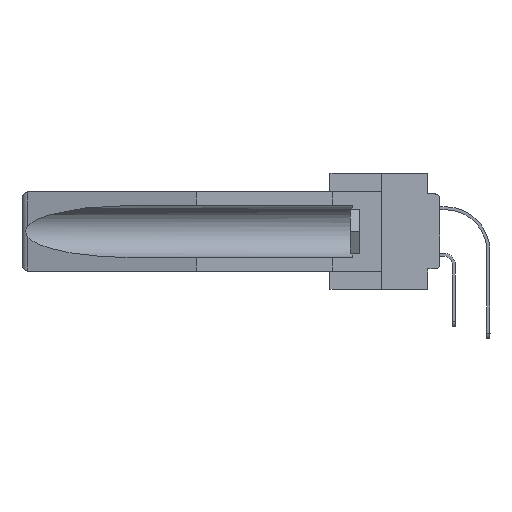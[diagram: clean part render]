
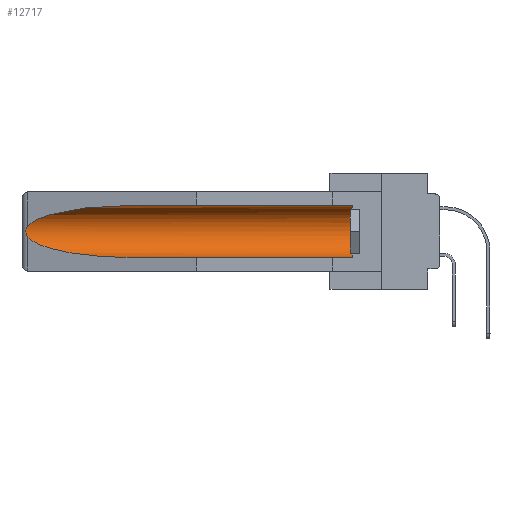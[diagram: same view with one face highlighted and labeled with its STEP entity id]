
A CAD part, left-side view. The second image highlights one B-rep face of the part: STEP entity #12717.
In plain terms, the highlighted cylindrical face has radius 2.857 mm (diameter 5.715 mm), a partial arc.
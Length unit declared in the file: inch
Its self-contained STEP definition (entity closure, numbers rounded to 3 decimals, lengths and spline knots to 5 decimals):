
#352 = VECTOR ( 'NONE', #33253, 39.37008 ) ;
#1443 = CARTESIAN_POINT ( 'NONE',  ( 0.155, -0.30754, -0.284 ) ) ;
#1604 = CARTESIAN_POINT ( 'NONE',  ( 0.2673, 1.5327, -0.16383 ) ) ;
#1840 = CARTESIAN_POINT ( 'NONE',  ( 0.21114, 1.30732, -0.059 ) ) ;
#2004 = CARTESIAN_POINT ( 'NONE',  ( 0.26537, 1.52718, -0.14972 ) ) ;
#2358 = FACE_OUTER_BOUND ( 'NONE', #9499, .T. ) ;
#2486 = CARTESIAN_POINT ( 'NONE',  ( 0.26537, 1.52718, -0.14972 ) ) ;
#6204 = CARTESIAN_POINT ( 'NONE',  ( 0.155, 0.126, -0.1715 ) ) ;
#7096 = AXIS2_PLACEMENT_3D ( 'NONE', #14625, #23836, #36127 ) ;
#7277 = LINE ( 'NONE', #1443, #23521 ) ;
#7539 = VERTEX_POINT ( 'NONE', #20993 ) ;
#7878 = VERTEX_POINT ( 'NONE', #8893 ) ;
#8505 = CARTESIAN_POINT ( 'NONE',  ( 0.155, -0.30754, -0.059 ) ) ;
#8737 = CARTESIAN_POINT ( 'NONE',  ( 0.26537, 1.52718, -0.19328 ) ) ;
#8789 = VERTEX_POINT ( 'NONE', #2486 ) ;
#8893 = CARTESIAN_POINT ( 'NONE',  ( 0.155, 1.07973, -0.284 ) ) ;
#9394 = ORIENTED_EDGE ( 'NONE', *, *, #31100, .T. ) ;
#9499 = EDGE_LOOP ( 'NONE', ( #32485, #18667, #29372, #27656, #9394, #21245 ) ) ;
#10788 = CARTESIAN_POINT ( 'NONE',  ( 0.25451, 1.48313, -0.24835 ) ) ;
#11075 = CARTESIAN_POINT ( 'NONE',  ( 0.26537, 1.52718, -0.14972 ) ) ;
#12717 = ADVANCED_FACE ( 'NONE', ( #2358 ), #29700, .F. ) ;
#14625 = CARTESIAN_POINT ( 'NONE',  ( 0.155, -0.30754, -0.1715 ) ) ;
#15066 = EDGE_CURVE ( 'NONE', #7539, #8789, #22315, .T. ) ;
#15300 = EDGE_CURVE ( 'NONE', #31904, #7878, #26425, .T. ) ;
#17088 = CARTESIAN_POINT ( 'NONE',  ( 0.26537, 1.52718, -0.19328 ) ) ;
#18108 = CARTESIAN_POINT ( 'NONE',  ( 0.155, 0.126, -0.059 ) ) ;
#18667 = ORIENTED_EDGE ( 'NONE', *, *, #24785, .T. ) ;
#19581 = CIRCLE ( 'NONE', #38325, 0.1125 ) ;
#20007 = CARTESIAN_POINT ( 'NONE',  ( 0.21114, 1.30732, -0.284 ) ) ;
#20078 = CARTESIAN_POINT ( 'NONE',  ( 0.26655, 1.53094, -0.18657 ) ) ;
#20220 = EDGE_CURVE ( 'NONE', #27734, #7539, #30629, .T. ) ;
#20993 = CARTESIAN_POINT ( 'NONE',  ( 0.155, 1.07973, -0.059 ) ) ;
#21245 = ORIENTED_EDGE ( 'NONE', *, *, #20220, .T. ) ;
#22315 =( BOUNDED_CURVE ( )  B_SPLINE_CURVE ( 3, ( #23315, #1840, #38634, #11075 ),
 .UNSPECIFIED., .F., .F. ) 
 B_SPLINE_CURVE_WITH_KNOTS ( ( 4, 4 ),
 ( 4.71239, 6.08839 ),
 .UNSPECIFIED. ) 
 CURVE ( )  GEOMETRIC_REPRESENTATION_ITEM ( )  RATIONAL_B_SPLINE_CURVE ( ( 1., 0.848, 0.848, 1. ) ) 
 REPRESENTATION_ITEM ( '' )  );
#23022 = VERTEX_POINT ( 'NONE', #26567 ) ;
#23095 = CARTESIAN_POINT ( 'NONE',  ( 0.26654, 1.53092, -0.15636 ) ) ;
#23315 = CARTESIAN_POINT ( 'NONE',  ( 0.155, 1.07973, -0.059 ) ) ;
#23521 = VECTOR ( 'NONE', #34643, 39.37008 ) ;
#23836 = DIRECTION ( 'NONE',  ( 0., 1., 0. ) ) ;
#24785 = EDGE_CURVE ( 'NONE', #8789, #31904, #27984, .T. ) ;
#25267 = DIRECTION ( 'NONE',  ( 0., -1., 0. ) ) ;
#26143 = CARTESIAN_POINT ( 'NONE',  ( 0.2673, 1.53269, -0.17917 ) ) ;
#26425 =( BOUNDED_CURVE ( )  B_SPLINE_CURVE ( 3, ( #38345, #10788, #20007, #35316 ),
 .UNSPECIFIED., .F., .T. ) 
 B_SPLINE_CURVE_WITH_KNOTS ( ( 4, 4 ),
 ( 0.1948, 1.5708 ),
 .UNSPECIFIED. ) 
 CURVE ( )  GEOMETRIC_REPRESENTATION_ITEM ( )  RATIONAL_B_SPLINE_CURVE ( ( 1., 0.848, 0.848, 1. ) ) 
 REPRESENTATION_ITEM ( '' )  );
#26528 = CARTESIAN_POINT ( 'NONE',  ( 0.2675, 1.53308, -0.16763 ) ) ;
#26567 = CARTESIAN_POINT ( 'NONE',  ( 0.155, 0.126, -0.284 ) ) ;
#27656 = ORIENTED_EDGE ( 'NONE', *, *, #32148, .F. ) ;
#27734 = VERTEX_POINT ( 'NONE', #18108 ) ;
#27984 = B_SPLINE_CURVE_WITH_KNOTS ( 'NONE', 3,
 ( #2004, #29151, #23095, #1604, #26528, #38801, #26143, #20078, #38418, #17088 ),
 .UNSPECIFIED., .F., .F.,
 ( 4, 2, 2, 2, 4 ),
 ( 0., 0.00029, 0.00058, 0.00087, 0.00117 ),
 .UNSPECIFIED. ) ;
#29151 = CARTESIAN_POINT ( 'NONE',  ( 0.26597, 1.52961, -0.15275 ) ) ;
#29372 = ORIENTED_EDGE ( 'NONE', *, *, #15300, .T. ) ;
#29700 = CYLINDRICAL_SURFACE ( 'NONE', #7096, 0.1125 ) ;
#30629 = LINE ( 'NONE', #8505, #352 ) ;
#30935 = DIRECTION ( 'NONE',  ( 0., 0., 1. ) ) ;
#31100 = EDGE_CURVE ( 'NONE', #23022, #27734, #19581, .T. ) ;
#31904 = VERTEX_POINT ( 'NONE', #8737 ) ;
#32148 = EDGE_CURVE ( 'NONE', #23022, #7878, #7277, .T. ) ;
#32485 = ORIENTED_EDGE ( 'NONE', *, *, #15066, .T. ) ;
#33253 = DIRECTION ( 'NONE',  ( 0., 1., 0. ) ) ;
#34643 = DIRECTION ( 'NONE',  ( 0., 1., 0. ) ) ;
#35316 = CARTESIAN_POINT ( 'NONE',  ( 0.155, 1.07973, -0.284 ) ) ;
#36127 = DIRECTION ( 'NONE',  ( 0., 0., 1. ) ) ;
#38325 = AXIS2_PLACEMENT_3D ( 'NONE', #6204, #25267, #30935 ) ;
#38345 = CARTESIAN_POINT ( 'NONE',  ( 0.26537, 1.52718, -0.19328 ) ) ;
#38418 = CARTESIAN_POINT ( 'NONE',  ( 0.26597, 1.5296, -0.19026 ) ) ;
#38634 = CARTESIAN_POINT ( 'NONE',  ( 0.25451, 1.48313, -0.09465 ) ) ;
#38801 = CARTESIAN_POINT ( 'NONE',  ( 0.2675, 1.53308, -0.17534 ) ) ;
